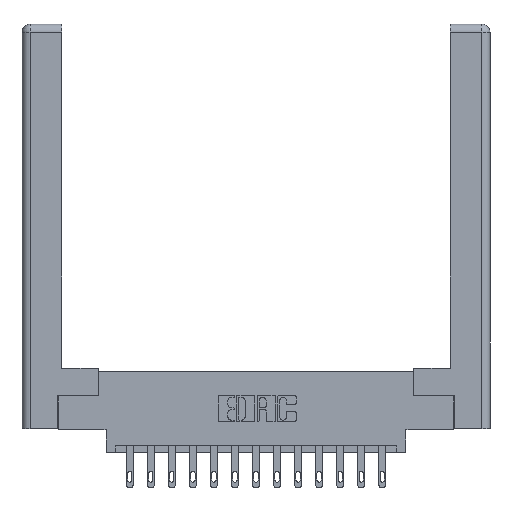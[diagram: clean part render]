
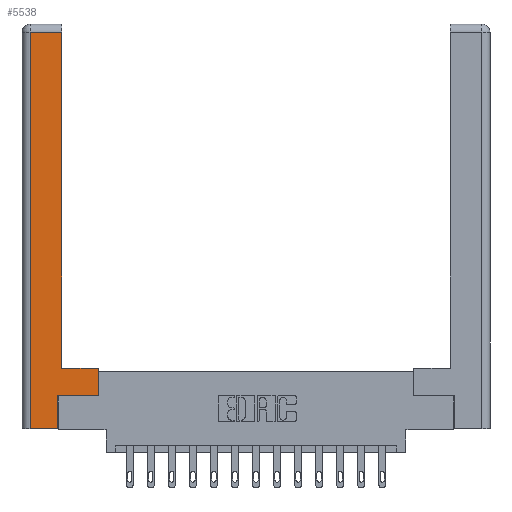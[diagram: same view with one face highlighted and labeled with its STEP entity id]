
A CAD part, top view. The second image highlights one B-rep face of the part: STEP entity #5538.
In plain terms, the highlighted planar face has unit normal (0, 0, 1).
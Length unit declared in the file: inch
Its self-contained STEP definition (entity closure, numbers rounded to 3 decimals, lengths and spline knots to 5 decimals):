
#259 = LINE ( 'NONE', #8575, #16061 ) ;
#269 = EDGE_CURVE ( 'NONE', #11633, #9601, #5175, .T. ) ;
#291 = VERTEX_POINT ( 'NONE', #815 ) ;
#587 = DIRECTION ( 'NONE',  ( 0., 0., -1. ) ) ;
#788 = VERTEX_POINT ( 'NONE', #7206 ) ;
#815 = CARTESIAN_POINT ( 'NONE',  ( 0.0615, 0., 0. ) ) ;
#1341 = EDGE_CURVE ( 'NONE', #13108, #11311, #6545, .T. ) ;
#1690 = EDGE_CURVE ( 'NONE', #11311, #11633, #9288, .T. ) ;
#1858 = VECTOR ( 'NONE', #7295, 39.37008 ) ;
#1869 = DIRECTION ( 'NONE',  ( 1., 0., 0. ) ) ;
#1926 = CARTESIAN_POINT ( 'NONE',  ( 0.265, 0., 0. ) ) ;
#1935 = CARTESIAN_POINT ( 'NONE',  ( 0., 0., 0. ) ) ;
#2906 = CARTESIAN_POINT ( 'NONE',  ( 0.565, 0.45, 0. ) ) ;
#3088 = AXIS2_PLACEMENT_3D ( 'NONE', #1935, #587, #10788 ) ;
#3134 = VECTOR ( 'NONE', #10714, 39.37008 ) ;
#3136 = VECTOR ( 'NONE', #14136, 39.37008 ) ;
#3165 = EDGE_CURVE ( 'NONE', #9601, #12640, #259, .T. ) ;
#3182 = ORIENTED_EDGE ( 'NONE', *, *, #5306, .T. ) ;
#3224 = DIRECTION ( 'NONE',  ( 0., 1., 0. ) ) ;
#3407 = ORIENTED_EDGE ( 'NONE', *, *, #269, .T. ) ;
#3982 = EDGE_CURVE ( 'NONE', #291, #788, #8030, .T. ) ;
#4847 = CARTESIAN_POINT ( 'NONE',  ( 0.295, 2.94, 0. ) ) ;
#5175 = LINE ( 'NONE', #13681, #8138 ) ;
#5196 = DIRECTION ( 'NONE',  ( 0., -1., 0. ) ) ;
#5306 = EDGE_CURVE ( 'NONE', #12640, #291, #13653, .T. ) ;
#5538 = ADVANCED_FACE ( 'NONE', ( #9881 ), #6967, .F. ) ;
#5837 = EDGE_CURVE ( 'NONE', #788, #10856, #13024, .T. ) ;
#5923 = CARTESIAN_POINT ( 'NONE',  ( 0.265, 0.245, 0. ) ) ;
#6069 = ORIENTED_EDGE ( 'NONE', *, *, #1341, .T. ) ;
#6545 = LINE ( 'NONE', #8270, #3134 ) ;
#6967 = PLANE ( 'NONE',  #3088 ) ;
#7206 = CARTESIAN_POINT ( 'NONE',  ( 0.265, 0., 0. ) ) ;
#7295 = DIRECTION ( 'NONE',  ( 1., 0., 0. ) ) ;
#7862 = CARTESIAN_POINT ( 'NONE',  ( 0.565, 0.245, 0. ) ) ;
#7882 = VECTOR ( 'NONE', #5196, 39.37008 ) ;
#8030 = LINE ( 'NONE', #1926, #1858 ) ;
#8138 = VECTOR ( 'NONE', #16412, 39.37008 ) ;
#8227 = ORIENTED_EDGE ( 'NONE', *, *, #3982, .T. ) ;
#8270 = CARTESIAN_POINT ( 'NONE',  ( 0.565, 0.45, 0. ) ) ;
#8277 = ORIENTED_EDGE ( 'NONE', *, *, #5837, .T. ) ;
#8348 = VECTOR ( 'NONE', #1869, 39.37008 ) ;
#8575 = CARTESIAN_POINT ( 'NONE',  ( 0.0615, 2.94, 0. ) ) ;
#9288 = LINE ( 'NONE', #11063, #3136 ) ;
#9601 = VERTEX_POINT ( 'NONE', #4847 ) ;
#9665 = VECTOR ( 'NONE', #3224, 39.37008 ) ;
#9818 = ORIENTED_EDGE ( 'NONE', *, *, #3165, .T. ) ;
#9881 = FACE_OUTER_BOUND ( 'NONE', #14499, .T. ) ;
#10470 = CARTESIAN_POINT ( 'NONE',  ( 0.0615, 2.94, 0. ) ) ;
#10656 = ORIENTED_EDGE ( 'NONE', *, *, #1690, .T. ) ;
#10714 = DIRECTION ( 'NONE',  ( 0., 1., 0. ) ) ;
#10788 = DIRECTION ( 'NONE',  ( -1., 0., 0. ) ) ;
#10856 = VERTEX_POINT ( 'NONE', #5923 ) ;
#11063 = CARTESIAN_POINT ( 'NONE',  ( 0.295, 0.45, 0. ) ) ;
#11311 = VERTEX_POINT ( 'NONE', #2906 ) ;
#11633 = VERTEX_POINT ( 'NONE', #14164 ) ;
#11697 = EDGE_CURVE ( 'NONE', #10856, #13108, #11726, .T. ) ;
#11726 = LINE ( 'NONE', #13386, #8348 ) ;
#12640 = VERTEX_POINT ( 'NONE', #10470 ) ;
#13024 = LINE ( 'NONE', #15988, #9665 ) ;
#13108 = VERTEX_POINT ( 'NONE', #7862 ) ;
#13386 = CARTESIAN_POINT ( 'NONE',  ( 0.565, 0.245, 0. ) ) ;
#13653 = LINE ( 'NONE', #15477, #7882 ) ;
#13681 = CARTESIAN_POINT ( 'NONE',  ( 0.295, 3., 0. ) ) ;
#13909 = ORIENTED_EDGE ( 'NONE', *, *, #11697, .T. ) ;
#13966 = DIRECTION ( 'NONE',  ( -1., 0., 0. ) ) ;
#14136 = DIRECTION ( 'NONE',  ( -1., 0., 0. ) ) ;
#14164 = CARTESIAN_POINT ( 'NONE',  ( 0.295, 0.45, 0. ) ) ;
#14499 = EDGE_LOOP ( 'NONE', ( #3407, #9818, #3182, #8227, #8277, #13909, #6069, #10656 ) ) ;
#15477 = CARTESIAN_POINT ( 'NONE',  ( 0.0615, 0., 0. ) ) ;
#15988 = CARTESIAN_POINT ( 'NONE',  ( 0.265, 0.245, 0. ) ) ;
#16061 = VECTOR ( 'NONE', #13966, 39.37008 ) ;
#16412 = DIRECTION ( 'NONE',  ( 0., 1., 0. ) ) ;
